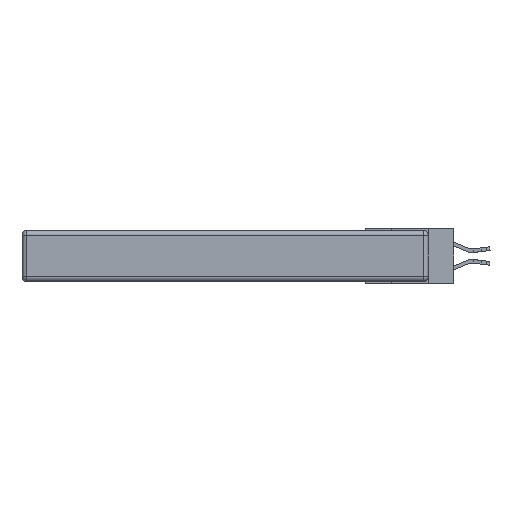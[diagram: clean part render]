
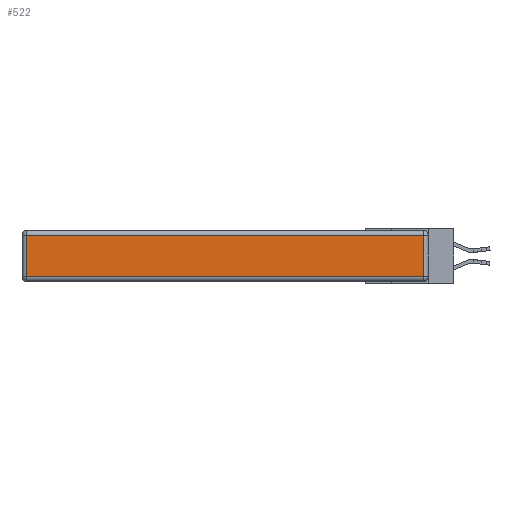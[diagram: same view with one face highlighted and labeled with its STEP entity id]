
A CAD part, left-side view. The second image highlights one B-rep face of the part: STEP entity #522.
In plain terms, the highlighted planar face has unit normal (-1, 0, 0).
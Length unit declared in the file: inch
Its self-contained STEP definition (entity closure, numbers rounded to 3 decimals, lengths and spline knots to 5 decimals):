
#522 = ADVANCED_FACE ( 'NONE', ( #7752 ), #3352, .T. ) ;
#784 = EDGE_CURVE ( 'NONE', #10238, #10318, #11385, .T. ) ;
#965 = ORIENTED_EDGE ( 'NONE', *, *, #3049, .T. ) ;
#1574 = VECTOR ( 'NONE', #9551, 39.37008 ) ;
#1755 = LINE ( 'NONE', #1793, #1574 ) ;
#1793 = CARTESIAN_POINT ( 'NONE',  ( 0., 0., -0.313 ) ) ;
#2212 = ORIENTED_EDGE ( 'NONE', *, *, #3962, .T. ) ;
#2976 = VECTOR ( 'NONE', #14575, 39.37008 ) ;
#3049 = EDGE_CURVE ( 'NONE', #10318, #3621, #3622, .T. ) ;
#3111 = CARTESIAN_POINT ( 'NONE',  ( 0., 0.03, -0.343 ) ) ;
#3352 = PLANE ( 'NONE',  #9299 ) ;
#3621 = VERTEX_POINT ( 'NONE', #8473 ) ;
#3622 = LINE ( 'NONE', #9134, #7810 ) ;
#3962 = EDGE_CURVE ( 'NONE', #13104, #10238, #1755, .T. ) ;
#4504 = CARTESIAN_POINT ( 'NONE',  ( 0., 0., -0.343 ) ) ;
#5329 = CARTESIAN_POINT ( 'NONE',  ( 0., 2.72, -0.343 ) ) ;
#5514 = CARTESIAN_POINT ( 'NONE',  ( 0., 0.03, -0.313 ) ) ;
#5545 = ORIENTED_EDGE ( 'NONE', *, *, #784, .T. ) ;
#5985 = EDGE_CURVE ( 'NONE', #3621, #13104, #14269, .T. ) ;
#6948 = ORIENTED_EDGE ( 'NONE', *, *, #5985, .T. ) ;
#7752 = FACE_OUTER_BOUND ( 'NONE', #11056, .T. ) ;
#7810 = VECTOR ( 'NONE', #10143, 39.37008 ) ;
#8473 = CARTESIAN_POINT ( 'NONE',  ( 0., 2.72, -0.03 ) ) ;
#9134 = CARTESIAN_POINT ( 'NONE',  ( 0., 2.75, -0.03 ) ) ;
#9299 = AXIS2_PLACEMENT_3D ( 'NONE', #4504, #12623, #14916 ) ;
#9551 = DIRECTION ( 'NONE',  ( 0., -1., 0. ) ) ;
#9890 = CARTESIAN_POINT ( 'NONE',  ( 0., 2.72, -0.313 ) ) ;
#10143 = DIRECTION ( 'NONE',  ( 0., 1., 0. ) ) ;
#10238 = VERTEX_POINT ( 'NONE', #5514 ) ;
#10318 = VERTEX_POINT ( 'NONE', #12677 ) ;
#11056 = EDGE_LOOP ( 'NONE', ( #2212, #5545, #965, #6948 ) ) ;
#11385 = LINE ( 'NONE', #3111, #14686 ) ;
#12623 = DIRECTION ( 'NONE',  ( -1., 0., 0. ) ) ;
#12677 = CARTESIAN_POINT ( 'NONE',  ( 0., 0.03, -0.03 ) ) ;
#13104 = VERTEX_POINT ( 'NONE', #9890 ) ;
#14269 = LINE ( 'NONE', #5329, #2976 ) ;
#14575 = DIRECTION ( 'NONE',  ( 0., 0., -1. ) ) ;
#14686 = VECTOR ( 'NONE', #14830, 39.37008 ) ;
#14830 = DIRECTION ( 'NONE',  ( 0., 0., 1. ) ) ;
#14916 = DIRECTION ( 'NONE',  ( 0., 0., 1. ) ) ;
